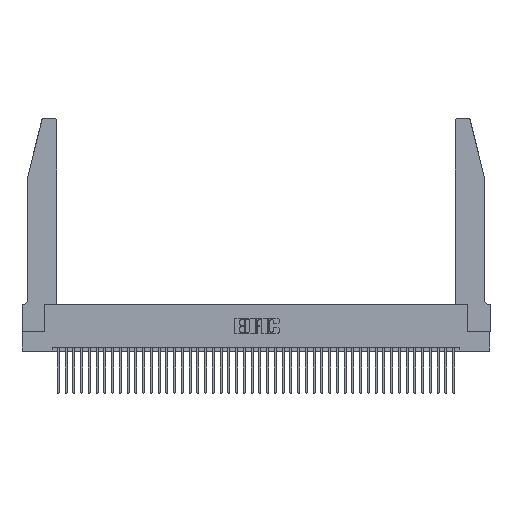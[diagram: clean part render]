
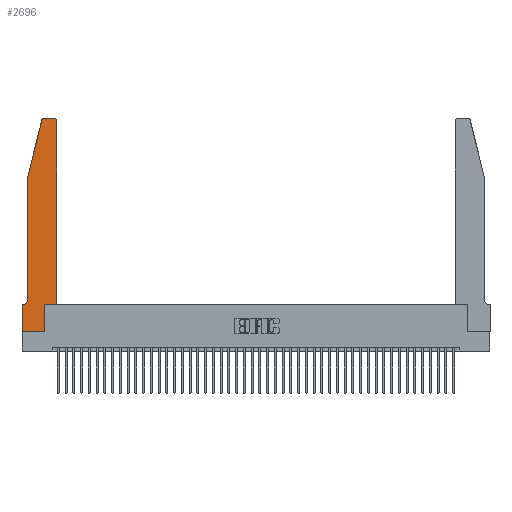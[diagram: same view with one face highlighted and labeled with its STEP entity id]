
A CAD part, top view. The second image highlights one B-rep face of the part: STEP entity #2696.
In plain terms, the highlighted planar face has unit normal (0, 0, 1).
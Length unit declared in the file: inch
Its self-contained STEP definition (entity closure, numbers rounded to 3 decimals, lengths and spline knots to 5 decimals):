
#46 = CARTESIAN_POINT ( 'NONE',  ( 0.0755, 2., 0.37 ) ) ;
#520 = EDGE_CURVE ( 'NONE', #2547, #4222, #10278, .T. ) ;
#750 = CARTESIAN_POINT ( 'NONE',  ( 0.2605, 2.75, 0.37 ) ) ;
#954 = ORIENTED_EDGE ( 'NONE', *, *, #32288, .T. ) ;
#1414 = AXIS2_PLACEMENT_3D ( 'NONE', #20186, #30169, #33647 ) ;
#1558 = ORIENTED_EDGE ( 'NONE', *, *, #17314, .T. ) ;
#1956 = VECTOR ( 'NONE', #32435, 39.37008 ) ;
#2547 = VERTEX_POINT ( 'NONE', #31101 ) ;
#2696 = ADVANCED_FACE ( 'NONE', ( #6424 ), #43458, .T. ) ;
#3225 = EDGE_CURVE ( 'NONE', #11669, #2547, #5336, .T. ) ;
#3571 = VERTEX_POINT ( 'NONE', #23397 ) ;
#4011 = CARTESIAN_POINT ( 'NONE',  ( 0.284, 2.75, 0.37 ) ) ;
#4157 = ORIENTED_EDGE ( 'NONE', *, *, #22778, .T. ) ;
#4222 = VERTEX_POINT ( 'NONE', #20838 ) ;
#4762 = DIRECTION ( 'NONE',  ( -1., 0., 0. ) ) ;
#5158 = EDGE_CURVE ( 'NONE', #3571, #12066, #31428, .T. ) ;
#5336 = CIRCLE ( 'NONE', #14828, 0.03 ) ;
#6424 = FACE_OUTER_BOUND ( 'NONE', #32749, .T. ) ;
#6658 = AXIS2_PLACEMENT_3D ( 'NONE', #28587, #25278, #4762 ) ;
#6674 = CARTESIAN_POINT ( 'NONE',  ( 0., 0., 0.37 ) ) ;
#6846 = VECTOR ( 'NONE', #18369, 39.37008 ) ;
#7072 = VECTOR ( 'NONE', #40422, 39.37008 ) ;
#7401 = CARTESIAN_POINT ( 'NONE',  ( 0.0755, 0.35, 0.37 ) ) ;
#7754 = ORIENTED_EDGE ( 'NONE', *, *, #27745, .T. ) ;
#7773 = EDGE_CURVE ( 'NONE', #32890, #43427, #28599, .T. ) ;
#8014 = VECTOR ( 'NONE', #34304, 39.37008 ) ;
#9032 = VERTEX_POINT ( 'NONE', #12236 ) ;
#9395 = DIRECTION ( 'NONE',  ( 1., 0., 0. ) ) ;
#10164 = ORIENTED_EDGE ( 'NONE', *, *, #43993, .T. ) ;
#10248 = CIRCLE ( 'NONE', #6658, 0.07 ) ;
#10278 = LINE ( 'NONE', #16121, #7072 ) ;
#10454 = LINE ( 'NONE', #6674, #1956 ) ;
#11669 = VERTEX_POINT ( 'NONE', #4011 ) ;
#11971 = VERTEX_POINT ( 'NONE', #39653 ) ;
#12066 = VERTEX_POINT ( 'NONE', #19925 ) ;
#12236 = CARTESIAN_POINT ( 'NONE',  ( 0.0755, 0.42, 0.37 ) ) ;
#12267 = VECTOR ( 'NONE', #33743, 39.37008 ) ;
#13425 = VECTOR ( 'NONE', #28296, 39.37008 ) ;
#13674 = ORIENTED_EDGE ( 'NONE', *, *, #34212, .T. ) ;
#14828 = AXIS2_PLACEMENT_3D ( 'NONE', #26055, #29977, #9395 ) ;
#15011 = VERTEX_POINT ( 'NONE', #18392 ) ;
#16121 = CARTESIAN_POINT ( 'NONE',  ( 0.0755, 2., 0.37 ) ) ;
#16884 = LINE ( 'NONE', #17428, #41570 ) ;
#17097 = CARTESIAN_POINT ( 'NONE',  ( 0.4505, 2.72, 0.37 ) ) ;
#17314 = EDGE_CURVE ( 'NONE', #36464, #11971, #30539, .T. ) ;
#17428 = CARTESIAN_POINT ( 'NONE',  ( 0.4505, 0.35, 0.37 ) ) ;
#17498 = LINE ( 'NONE', #28150, #6846 ) ;
#18369 = DIRECTION ( 'NONE',  ( 0., 1., 0. ) ) ;
#18392 = CARTESIAN_POINT ( 'NONE',  ( 0.0055, 0.35, 0.37 ) ) ;
#19925 = CARTESIAN_POINT ( 'NONE',  ( 0.2865, 0.35, 0.37 ) ) ;
#20186 = CARTESIAN_POINT ( 'NONE',  ( 0., 0.35, 0.37 ) ) ;
#20453 = ORIENTED_EDGE ( 'NONE', *, *, #520, .T. ) ;
#20480 = EDGE_CURVE ( 'NONE', #43427, #11669, #22579, .T. ) ;
#20838 = CARTESIAN_POINT ( 'NONE',  ( 0.0755, 2., 0.37 ) ) ;
#21495 = ORIENTED_EDGE ( 'NONE', *, *, #3225, .T. ) ;
#22579 = LINE ( 'NONE', #750, #13425 ) ;
#22778 = EDGE_CURVE ( 'NONE', #15011, #36464, #28356, .T. ) ;
#23397 = CARTESIAN_POINT ( 'NONE',  ( 0.2865, 0., 0.37 ) ) ;
#23712 = DIRECTION ( 'NONE',  ( 0., 0., 1. ) ) ;
#23758 = CARTESIAN_POINT ( 'NONE',  ( 0., 0., 0.37 ) ) ;
#24332 = ORIENTED_EDGE ( 'NONE', *, *, #42797, .T. ) ;
#25278 = DIRECTION ( 'NONE',  ( 0., 0., -1. ) ) ;
#26055 = CARTESIAN_POINT ( 'NONE',  ( 0.284, 2.72, 0.37 ) ) ;
#26595 = CARTESIAN_POINT ( 'NONE',  ( 0., 0.35, 0.37 ) ) ;
#27279 = CARTESIAN_POINT ( 'NONE',  ( 0.4505, 0.35, 0.37 ) ) ;
#27373 = LINE ( 'NONE', #46, #8014 ) ;
#27683 = DIRECTION ( 'NONE',  ( 1., 0., 0. ) ) ;
#27745 = EDGE_CURVE ( 'NONE', #11971, #3571, #10454, .T. ) ;
#28150 = CARTESIAN_POINT ( 'NONE',  ( 0.4505, 0.35, 0.37 ) ) ;
#28296 = DIRECTION ( 'NONE',  ( -1., 0., 0. ) ) ;
#28356 = LINE ( 'NONE', #7401, #37998 ) ;
#28587 = CARTESIAN_POINT ( 'NONE',  ( 0.0055, 0.42, 0.37 ) ) ;
#28599 = CIRCLE ( 'NONE', #44173, 0.03 ) ;
#29977 = DIRECTION ( 'NONE',  ( 0., 0., 1. ) ) ;
#30118 = ORIENTED_EDGE ( 'NONE', *, *, #7773, .T. ) ;
#30169 = DIRECTION ( 'NONE',  ( 0., 0., 1. ) ) ;
#30334 = DIRECTION ( 'NONE',  ( 0., 1., 0. ) ) ;
#30509 = DIRECTION ( 'NONE',  ( 1., 0., 0. ) ) ;
#30539 = LINE ( 'NONE', #23758, #12267 ) ;
#30956 = CARTESIAN_POINT ( 'NONE',  ( 0.2865, 0.35, 0.37 ) ) ;
#30983 = ORIENTED_EDGE ( 'NONE', *, *, #20480, .T. ) ;
#31101 = CARTESIAN_POINT ( 'NONE',  ( 0.25487, 2.72718, 0.37 ) ) ;
#31428 = LINE ( 'NONE', #30956, #36822 ) ;
#32288 = EDGE_CURVE ( 'NONE', #12066, #37059, #16884, .T. ) ;
#32435 = DIRECTION ( 'NONE',  ( 1., 0., 0. ) ) ;
#32749 = EDGE_LOOP ( 'NONE', ( #30983, #21495, #20453, #24332, #13674, #4157, #1558, #7754, #35533, #954, #10164, #30118 ) ) ;
#32890 = VERTEX_POINT ( 'NONE', #17097 ) ;
#33515 = DIRECTION ( 'NONE',  ( -1., 0., 0. ) ) ;
#33647 = DIRECTION ( 'NONE',  ( 1., 0., 0. ) ) ;
#33678 = CARTESIAN_POINT ( 'NONE',  ( 0.4205, 2.72, 0.37 ) ) ;
#33743 = DIRECTION ( 'NONE',  ( 0., -1., 0. ) ) ;
#34212 = EDGE_CURVE ( 'NONE', #9032, #15011, #10248, .T. ) ;
#34304 = DIRECTION ( 'NONE',  ( 0., -1., 0. ) ) ;
#35533 = ORIENTED_EDGE ( 'NONE', *, *, #5158, .T. ) ;
#36464 = VERTEX_POINT ( 'NONE', #26595 ) ;
#36822 = VECTOR ( 'NONE', #30334, 39.37008 ) ;
#37059 = VERTEX_POINT ( 'NONE', #27279 ) ;
#37412 = CARTESIAN_POINT ( 'NONE',  ( 0.4205, 2.75, 0.37 ) ) ;
#37998 = VECTOR ( 'NONE', #33515, 39.37008 ) ;
#39653 = CARTESIAN_POINT ( 'NONE',  ( 0., 0., 0.37 ) ) ;
#40422 = DIRECTION ( 'NONE',  ( -0.239, -0.971, 0. ) ) ;
#41570 = VECTOR ( 'NONE', #27683, 39.37008 ) ;
#42797 = EDGE_CURVE ( 'NONE', #4222, #9032, #27373, .T. ) ;
#43427 = VERTEX_POINT ( 'NONE', #37412 ) ;
#43458 = PLANE ( 'NONE',  #1414 ) ;
#43993 = EDGE_CURVE ( 'NONE', #37059, #32890, #17498, .T. ) ;
#44173 = AXIS2_PLACEMENT_3D ( 'NONE', #33678, #23712, #30509 ) ;
